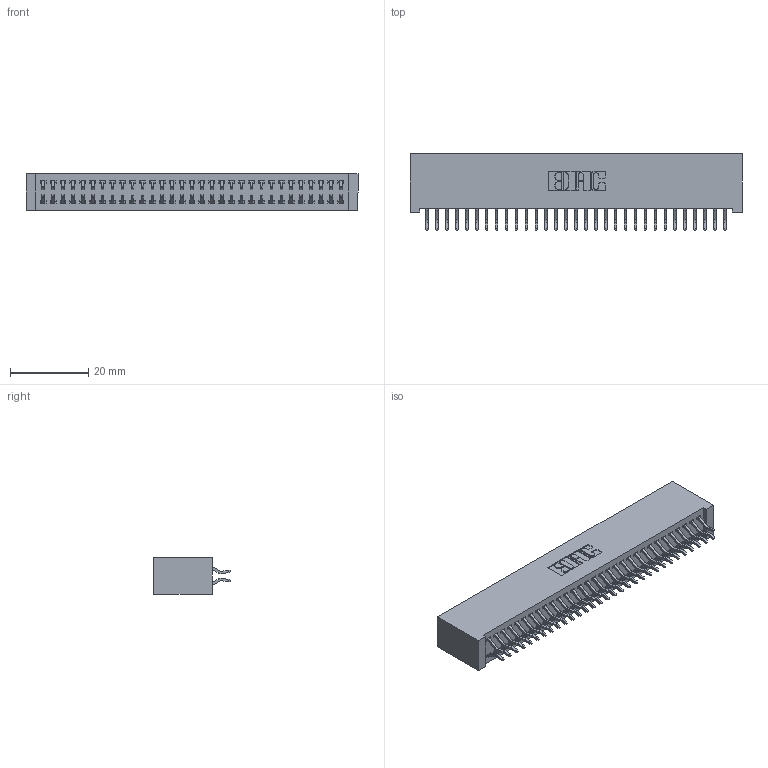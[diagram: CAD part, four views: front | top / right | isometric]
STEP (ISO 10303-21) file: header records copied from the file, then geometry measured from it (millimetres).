
FILE_DESCRIPTION (( 'STEP AP203' ), '1' );
FILE_NAME ('392-062-556-201.STEP', '2018-08-17T21:16:26', ( '' ), ( '' ), 'SwSTEP 2.0', 'SolidWorks 2016', '' );
FILE_SCHEMA (( 'CONFIG_CONTROL_DESIGN' ));
Length unit declared in the file: inch
Products named in the file (3): 342 Part_Lugless; 345-292-001_556 Tail; 392-062-556-201
Assembly tree (63 placements, depth 2):
  392-062-556-201
    342 Part_Lugless
    345-292-001_556 Tail  x62
Bounding box: 84.99 x 19.58 x 9.4 mm (x, y, z)
Volume: 8022.1 mm3; surface area: 13173 mm2
Topology: 63 solids, 63 shells, 3698 faces, 11001 edges, 7250 vertices
Faces by surface type: plane 2542, cylinder 1156
Entity records: 21177 total; most frequent: CARTESIAN_POINT 3534, ORIENTED_EDGE 3458, DIRECTION 3021, EDGE_CURVE 1729, LINE 1601, VECTOR 1601, VERTEX_POINT 1150, AXIS2_PLACEMENT_3D 710
